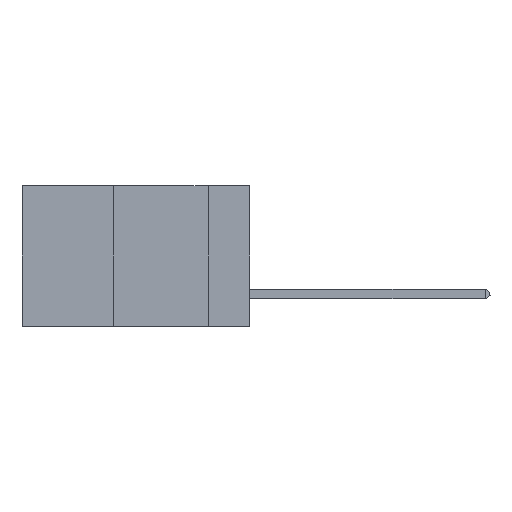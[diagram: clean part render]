
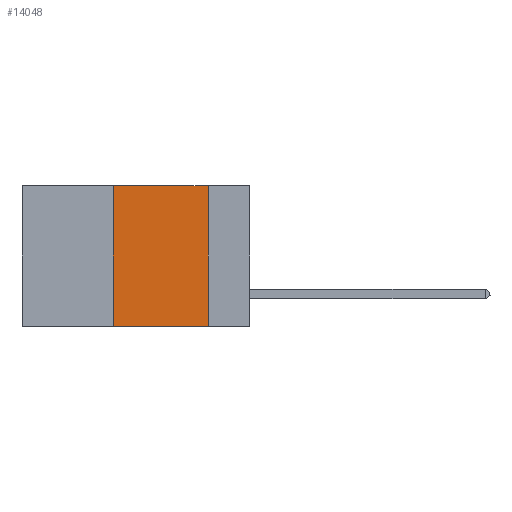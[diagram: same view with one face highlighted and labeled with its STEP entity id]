
A CAD part, left-side view. The second image highlights one B-rep face of the part: STEP entity #14048.
In plain terms, the highlighted planar face has unit normal (-1, 0, 0).
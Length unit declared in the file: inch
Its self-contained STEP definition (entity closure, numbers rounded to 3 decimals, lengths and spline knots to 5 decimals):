
#629 = DIRECTION ( 'NONE',  ( 0., -1., 0. ) ) ;
#996 = PLANE ( 'NONE',  #3468 ) ;
#1676 = LINE ( 'NONE', #4281, #10564 ) ;
#2822 = ORIENTED_EDGE ( 'NONE', *, *, #5696, .F. ) ;
#3468 = AXIS2_PLACEMENT_3D ( 'NONE', #6651, #4233, #12286 ) ;
#3917 = VECTOR ( 'NONE', #6949, 39.37008 ) ;
#3963 = CARTESIAN_POINT ( 'NONE',  ( 0., 0.6, -0.37 ) ) ;
#3984 = CARTESIAN_POINT ( 'NONE',  ( 0., 0.11, 0. ) ) ;
#3997 = EDGE_CURVE ( 'NONE', #13489, #10277, #10619, .T. ) ;
#4209 = EDGE_CURVE ( 'NONE', #4802, #10277, #9581, .T. ) ;
#4233 = DIRECTION ( 'NONE',  ( 1., 0., 0. ) ) ;
#4281 = CARTESIAN_POINT ( 'NONE',  ( 0., 0.36, 0. ) ) ;
#4802 = VERTEX_POINT ( 'NONE', #12811 ) ;
#5696 = EDGE_CURVE ( 'NONE', #4802, #11341, #1676, .T. ) ;
#6173 = ORIENTED_EDGE ( 'NONE', *, *, #4209, .T. ) ;
#6651 = CARTESIAN_POINT ( 'NONE',  ( 0., 0.6, 0. ) ) ;
#6949 = DIRECTION ( 'NONE',  ( 0., -1., 0. ) ) ;
#8731 = FACE_OUTER_BOUND ( 'NONE', #12551, .T. ) ;
#9168 = ORIENTED_EDGE ( 'NONE', *, *, #3997, .F. ) ;
#9230 = VECTOR ( 'NONE', #10093, 39.37008 ) ;
#9440 = CARTESIAN_POINT ( 'NONE',  ( 0., 0.11, 0. ) ) ;
#9581 = LINE ( 'NONE', #3963, #12833 ) ;
#10093 = DIRECTION ( 'NONE',  ( 0., 0., -1. ) ) ;
#10202 = LINE ( 'NONE', #12329, #3917 ) ;
#10277 = VERTEX_POINT ( 'NONE', #13380 ) ;
#10564 = VECTOR ( 'NONE', #14239, 39.37008 ) ;
#10619 = LINE ( 'NONE', #9440, #9230 ) ;
#11341 = VERTEX_POINT ( 'NONE', #13710 ) ;
#12286 = DIRECTION ( 'NONE',  ( 0., 0., -1. ) ) ;
#12329 = CARTESIAN_POINT ( 'NONE',  ( 0., 0.6, 0. ) ) ;
#12461 = EDGE_CURVE ( 'NONE', #11341, #13489, #10202, .T. ) ;
#12551 = EDGE_LOOP ( 'NONE', ( #9168, #13625, #2822, #6173 ) ) ;
#12811 = CARTESIAN_POINT ( 'NONE',  ( 0., 0.36, -0.37 ) ) ;
#12833 = VECTOR ( 'NONE', #629, 39.37008 ) ;
#13380 = CARTESIAN_POINT ( 'NONE',  ( 0., 0.11, -0.37 ) ) ;
#13489 = VERTEX_POINT ( 'NONE', #3984 ) ;
#13625 = ORIENTED_EDGE ( 'NONE', *, *, #12461, .F. ) ;
#13710 = CARTESIAN_POINT ( 'NONE',  ( 0., 0.36, 0. ) ) ;
#14048 = ADVANCED_FACE ( 'NONE', ( #8731 ), #996, .F. ) ;
#14239 = DIRECTION ( 'NONE',  ( 0., 0., 1. ) ) ;
